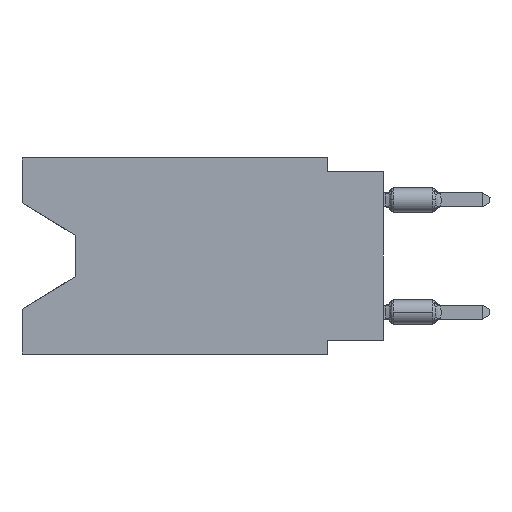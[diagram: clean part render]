
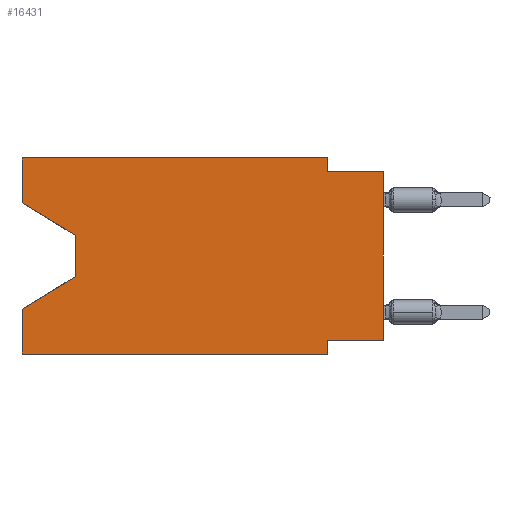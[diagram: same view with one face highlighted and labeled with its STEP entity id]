
A CAD part, left-side view. The second image highlights one B-rep face of the part: STEP entity #16431.
In plain terms, the highlighted planar face has unit normal (-1, 0, 0).
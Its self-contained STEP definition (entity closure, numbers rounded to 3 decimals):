
#419 = LINE ( 'NONE', #56406, #27894 ) ;
#838 = CARTESIAN_POINT ( 'NONE',  ( 0., 2.54, -0.635 ) ) ;
#894 = ORIENTED_EDGE ( 'NONE', *, *, #21293, .F. ) ;
#941 = EDGE_CURVE ( 'NONE', #37239, #10818, #60193, .T. ) ;
#977 = DIRECTION ( 'NONE',  ( 0., 1., 0. ) ) ;
#1384 = CARTESIAN_POINT ( 'NONE',  ( 0., 2.54, -8.89 ) ) ;
#2252 = ORIENTED_EDGE ( 'NONE', *, *, #58212, .F. ) ;
#2742 = VERTEX_POINT ( 'NONE', #57600 ) ;
#4067 = VERTEX_POINT ( 'NONE', #30873 ) ;
#4111 = LINE ( 'NONE', #61015, #16162 ) ;
#4307 = VECTOR ( 'NONE', #48976, 1000. ) ;
#4727 = CARTESIAN_POINT ( 'NONE',  ( 0., 16.383, 0. ) ) ;
#5328 = LINE ( 'NONE', #15262, #12172 ) ;
#6345 = EDGE_CURVE ( 'NONE', #51267, #23810, #419, .T. ) ;
#7074 = LINE ( 'NONE', #53098, #35543 ) ;
#8585 = LINE ( 'NONE', #13242, #40163 ) ;
#9753 = VERTEX_POINT ( 'NONE', #4727 ) ;
#10075 = ORIENTED_EDGE ( 'NONE', *, *, #37023, .T. ) ;
#10655 = ORIENTED_EDGE ( 'NONE', *, *, #6345, .T. ) ;
#10818 = VERTEX_POINT ( 'NONE', #12491 ) ;
#11169 = ORIENTED_EDGE ( 'NONE', *, *, #33404, .F. ) ;
#11726 = DIRECTION ( 'NONE',  ( 0., 0., -1. ) ) ;
#11748 = EDGE_CURVE ( 'NONE', #4067, #9753, #21596, .T. ) ;
#12172 = VECTOR ( 'NONE', #977, 1000. ) ;
#12264 = LINE ( 'NONE', #39644, #4307 ) ;
#12320 = VERTEX_POINT ( 'NONE', #37367 ) ;
#12491 = CARTESIAN_POINT ( 'NONE',  ( 0., 16.383, -6.852 ) ) ;
#13126 = DIRECTION ( 'NONE',  ( 0., -1., 0. ) ) ;
#13242 = CARTESIAN_POINT ( 'NONE',  ( 0., 16.383, -8.89 ) ) ;
#15154 = DIRECTION ( 'NONE',  ( 0., 0., 1. ) ) ;
#15262 = CARTESIAN_POINT ( 'NONE',  ( 0., 0., -8.255 ) ) ;
#15455 = ORIENTED_EDGE ( 'NONE', *, *, #49120, .T. ) ;
#15992 = VERTEX_POINT ( 'NONE', #55031 ) ;
#16162 = VECTOR ( 'NONE', #21847, 1000. ) ;
#16431 = ADVANCED_FACE ( 'NONE', ( #21363 ), #26031, .F. ) ;
#16432 = ORIENTED_EDGE ( 'NONE', *, *, #11748, .F. ) ;
#18353 = VECTOR ( 'NONE', #43824, 1000. ) ;
#18457 = DIRECTION ( 'NONE',  ( 0., 0., 1. ) ) ;
#21293 = EDGE_CURVE ( 'NONE', #2742, #10818, #7074, .T. ) ;
#21363 = FACE_OUTER_BOUND ( 'NONE', #57201, .T. ) ;
#21596 = LINE ( 'NONE', #36835, #32877 ) ;
#21847 = DIRECTION ( 'NONE',  ( 0., -0.855, -0.519 ) ) ;
#23810 = VERTEX_POINT ( 'NONE', #35736 ) ;
#25358 = CARTESIAN_POINT ( 'NONE',  ( 0., 2.54, -8.89 ) ) ;
#25762 = LINE ( 'NONE', #40070, #31712 ) ;
#26031 = PLANE ( 'NONE',  #60916 ) ;
#27249 = DIRECTION ( 'NONE',  ( 0., 0.855, -0.519 ) ) ;
#27894 = VECTOR ( 'NONE', #18457, 1000. ) ;
#28952 = EDGE_CURVE ( 'NONE', #61434, #23810, #40803, .T. ) ;
#30477 = CARTESIAN_POINT ( 'NONE',  ( 0., 13.97, -3.505 ) ) ;
#30873 = CARTESIAN_POINT ( 'NONE',  ( 0., 16.383, -2.038 ) ) ;
#31308 = ORIENTED_EDGE ( 'NONE', *, *, #28952, .F. ) ;
#31516 = VECTOR ( 'NONE', #27249, 1000. ) ;
#31712 = VECTOR ( 'NONE', #54363, 1000. ) ;
#32312 = ORIENTED_EDGE ( 'NONE', *, *, #34634, .T. ) ;
#32877 = VECTOR ( 'NONE', #40568, 1000. ) ;
#33404 = EDGE_CURVE ( 'NONE', #9753, #15992, #12264, .T. ) ;
#34634 = EDGE_CURVE ( 'NONE', #2742, #38725, #8585, .T. ) ;
#35543 = VECTOR ( 'NONE', #15154, 1000. ) ;
#35736 = CARTESIAN_POINT ( 'NONE',  ( 0., 0., -0.635 ) ) ;
#36835 = CARTESIAN_POINT ( 'NONE',  ( 0., 16.383, 0. ) ) ;
#37023 = EDGE_CURVE ( 'NONE', #40589, #37239, #53165, .T. ) ;
#37239 = VERTEX_POINT ( 'NONE', #41938 ) ;
#37367 = CARTESIAN_POINT ( 'NONE',  ( 0., 2.54, -8.255 ) ) ;
#37667 = VECTOR ( 'NONE', #13126, 1000. ) ;
#38725 = VERTEX_POINT ( 'NONE', #25358 ) ;
#39644 = CARTESIAN_POINT ( 'NONE',  ( 0., 16.383, 0. ) ) ;
#40070 = CARTESIAN_POINT ( 'NONE',  ( 0., 2.54, 0. ) ) ;
#40163 = VECTOR ( 'NONE', #42148, 1000. ) ;
#40568 = DIRECTION ( 'NONE',  ( 0., 0., 1. ) ) ;
#40589 = VERTEX_POINT ( 'NONE', #41446 ) ;
#40803 = LINE ( 'NONE', #46404, #37667 ) ;
#40949 = DIRECTION ( 'NONE',  ( 1., 0., 0. ) ) ;
#41386 = EDGE_CURVE ( 'NONE', #15992, #61434, #25762, .T. ) ;
#41388 = ORIENTED_EDGE ( 'NONE', *, *, #41386, .F. ) ;
#41446 = CARTESIAN_POINT ( 'NONE',  ( 0., 13.97, -3.505 ) ) ;
#41938 = CARTESIAN_POINT ( 'NONE',  ( 0., 13.97, -5.385 ) ) ;
#42148 = DIRECTION ( 'NONE',  ( 0., -1., 0. ) ) ;
#42640 = EDGE_CURVE ( 'NONE', #12320, #38725, #43944, .T. ) ;
#43824 = DIRECTION ( 'NONE',  ( 0., 0., -1. ) ) ;
#43944 = LINE ( 'NONE', #1384, #51699 ) ;
#46404 = CARTESIAN_POINT ( 'NONE',  ( 0., 0., -0.635 ) ) ;
#48734 = CARTESIAN_POINT ( 'NONE',  ( 0., 0., -8.255 ) ) ;
#48976 = DIRECTION ( 'NONE',  ( 0., -1., 0. ) ) ;
#49120 = EDGE_CURVE ( 'NONE', #4067, #40589, #4111, .T. ) ;
#50877 = CARTESIAN_POINT ( 'NONE',  ( 0., 13.97, -5.385 ) ) ;
#51267 = VERTEX_POINT ( 'NONE', #48734 ) ;
#51699 = VECTOR ( 'NONE', #55458, 1000. ) ;
#53098 = CARTESIAN_POINT ( 'NONE',  ( 0., 16.383, 0. ) ) ;
#53165 = LINE ( 'NONE', #30477, #18353 ) ;
#53271 = ORIENTED_EDGE ( 'NONE', *, *, #42640, .F. ) ;
#54363 = DIRECTION ( 'NONE',  ( 0., 0., -1. ) ) ;
#55031 = CARTESIAN_POINT ( 'NONE',  ( 0., 2.54, 0. ) ) ;
#55261 = CARTESIAN_POINT ( 'NONE',  ( 0., 16.383, 0. ) ) ;
#55458 = DIRECTION ( 'NONE',  ( 0., 0., -1. ) ) ;
#56406 = CARTESIAN_POINT ( 'NONE',  ( 0., 0., 0. ) ) ;
#56537 = ORIENTED_EDGE ( 'NONE', *, *, #941, .T. ) ;
#57201 = EDGE_LOOP ( 'NONE', ( #15455, #10075, #56537, #894, #32312, #53271, #2252, #10655, #31308, #41388, #11169, #16432 ) ) ;
#57600 = CARTESIAN_POINT ( 'NONE',  ( 0., 16.383, -8.89 ) ) ;
#58212 = EDGE_CURVE ( 'NONE', #51267, #12320, #5328, .T. ) ;
#60193 = LINE ( 'NONE', #50877, #31516 ) ;
#60916 = AXIS2_PLACEMENT_3D ( 'NONE', #55261, #40949, #11726 ) ;
#61015 = CARTESIAN_POINT ( 'NONE',  ( 0., 16.383, -2.038 ) ) ;
#61434 = VERTEX_POINT ( 'NONE', #838 ) ;
